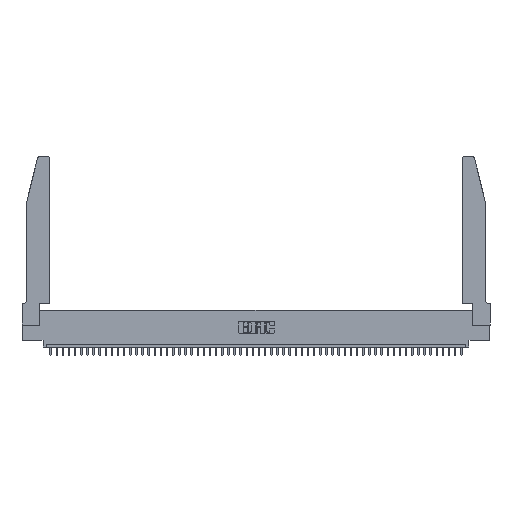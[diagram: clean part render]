
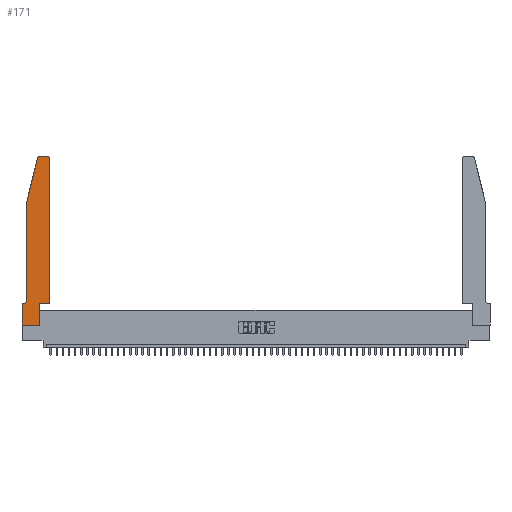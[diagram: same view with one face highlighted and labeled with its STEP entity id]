
A CAD part, top view. The second image highlights one B-rep face of the part: STEP entity #171.
In plain terms, the highlighted planar face has unit normal (0, 0, 1).
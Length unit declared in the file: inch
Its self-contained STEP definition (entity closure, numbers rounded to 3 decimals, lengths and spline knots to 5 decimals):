
#13 = ORIENTED_EDGE ( 'NONE', *, *, #20485, .T. ) ;
#171 = ADVANCED_FACE ( 'NONE', ( #5530 ), #13659, .T. ) ;
#1141 = ORIENTED_EDGE ( 'NONE', *, *, #18032, .T. ) ;
#1325 = CARTESIAN_POINT ( 'NONE',  ( 0., 0., 0.37 ) ) ;
#1405 = CARTESIAN_POINT ( 'NONE',  ( 0.2865, 0.35, 0.37 ) ) ;
#1880 = CARTESIAN_POINT ( 'NONE',  ( 0.4205, 2.75, 0.37 ) ) ;
#2229 = VECTOR ( 'NONE', #12704, 39.37008 ) ;
#2287 = CARTESIAN_POINT ( 'NONE',  ( 0.25487, 2.72718, 0.37 ) ) ;
#2716 = DIRECTION ( 'NONE',  ( 1., 0., 0. ) ) ;
#3330 = VECTOR ( 'NONE', #49036, 39.37008 ) ;
#3347 = EDGE_CURVE ( 'NONE', #30168, #31658, #4534, .T. ) ;
#4101 = LINE ( 'NONE', #18395, #52424 ) ;
#4330 = LINE ( 'NONE', #1405, #24577 ) ;
#4534 = LINE ( 'NONE', #32354, #3330 ) ;
#4567 = CARTESIAN_POINT ( 'NONE',  ( 0.0755, 0.42, 0.37 ) ) ;
#4757 = DIRECTION ( 'NONE',  ( 1., 0., 0. ) ) ;
#4932 = LINE ( 'NONE', #9479, #21395 ) ;
#5530 = FACE_OUTER_BOUND ( 'NONE', #16073, .T. ) ;
#5671 = CARTESIAN_POINT ( 'NONE',  ( 0., 0.35, 0.37 ) ) ;
#6887 = CARTESIAN_POINT ( 'NONE',  ( 0.4505, 0.35, 0.37 ) ) ;
#7756 = LINE ( 'NONE', #6887, #33646 ) ;
#8350 = AXIS2_PLACEMENT_3D ( 'NONE', #5671, #14010, #30314 ) ;
#8376 = CIRCLE ( 'NONE', #36357, 0.03 ) ;
#8532 = CARTESIAN_POINT ( 'NONE',  ( 0.4205, 2.72, 0.37 ) ) ;
#8862 = EDGE_CURVE ( 'NONE', #36129, #30168, #27700, .T. ) ;
#9057 = DIRECTION ( 'NONE',  ( 0., 0., -1. ) ) ;
#9324 = EDGE_CURVE ( 'NONE', #16800, #15200, #37878, .T. ) ;
#9479 = CARTESIAN_POINT ( 'NONE',  ( 0.4505, 0.35, 0.37 ) ) ;
#9498 = CARTESIAN_POINT ( 'NONE',  ( 0.284, 2.75, 0.37 ) ) ;
#9844 = CARTESIAN_POINT ( 'NONE',  ( 0., 0.35, 0.37 ) ) ;
#11796 = VERTEX_POINT ( 'NONE', #40973 ) ;
#12537 = CARTESIAN_POINT ( 'NONE',  ( 0.0755, 2., 0.37 ) ) ;
#12704 = DIRECTION ( 'NONE',  ( -0.239, -0.971, 0. ) ) ;
#12816 = EDGE_CURVE ( 'NONE', #49598, #34882, #16772, .T. ) ;
#13659 = PLANE ( 'NONE',  #8350 ) ;
#14010 = DIRECTION ( 'NONE',  ( 0., 0., 1. ) ) ;
#14015 = ORIENTED_EDGE ( 'NONE', *, *, #25178, .T. ) ;
#14162 = DIRECTION ( 'NONE',  ( 0., -1., 0. ) ) ;
#14476 = DIRECTION ( 'NONE',  ( 1., 0., 0. ) ) ;
#15200 = VERTEX_POINT ( 'NONE', #1880 ) ;
#15762 = CIRCLE ( 'NONE', #35798, 0.07 ) ;
#16073 = EDGE_LOOP ( 'NONE', ( #1141, #28969, #47659, #48011, #13, #52396, #35775, #38421, #27504, #38882, #14015, #41162 ) ) ;
#16536 = LINE ( 'NONE', #1325, #35635 ) ;
#16772 = LINE ( 'NONE', #12537, #2229 ) ;
#16800 = VERTEX_POINT ( 'NONE', #46149 ) ;
#17211 = EDGE_CURVE ( 'NONE', #19001, #30820, #4330, .T. ) ;
#18032 = EDGE_CURVE ( 'NONE', #15200, #28857, #52316, .T. ) ;
#18395 = CARTESIAN_POINT ( 'NONE',  ( 0.0755, 2., 0.37 ) ) ;
#19001 = VERTEX_POINT ( 'NONE', #19249 ) ;
#19249 = CARTESIAN_POINT ( 'NONE',  ( 0.2865, 0., 0.37 ) ) ;
#20126 = AXIS2_PLACEMENT_3D ( 'NONE', #8532, #29008, #4757 ) ;
#20485 = EDGE_CURVE ( 'NONE', #28073, #36129, #15762, .T. ) ;
#20636 = CARTESIAN_POINT ( 'NONE',  ( 0., 0., 0.37 ) ) ;
#21395 = VECTOR ( 'NONE', #50297, 39.37008 ) ;
#24577 = VECTOR ( 'NONE', #49690, 39.37008 ) ;
#25178 = EDGE_CURVE ( 'NONE', #11796, #16800, #4932, .T. ) ;
#25651 = CARTESIAN_POINT ( 'NONE',  ( 0.284, 2.72, 0.37 ) ) ;
#27504 = ORIENTED_EDGE ( 'NONE', *, *, #17211, .T. ) ;
#27700 = LINE ( 'NONE', #36387, #48770 ) ;
#27783 = DIRECTION ( 'NONE',  ( -1., 0., 0. ) ) ;
#28073 = VERTEX_POINT ( 'NONE', #4567 ) ;
#28617 = VECTOR ( 'NONE', #50097, 39.37008 ) ;
#28857 = VERTEX_POINT ( 'NONE', #9498 ) ;
#28969 = ORIENTED_EDGE ( 'NONE', *, *, #29483, .T. ) ;
#29008 = DIRECTION ( 'NONE',  ( 0., 0., 1. ) ) ;
#29483 = EDGE_CURVE ( 'NONE', #28857, #49598, #8376, .T. ) ;
#30168 = VERTEX_POINT ( 'NONE', #9844 ) ;
#30314 = DIRECTION ( 'NONE',  ( 1., 0., 0. ) ) ;
#30820 = VERTEX_POINT ( 'NONE', #33991 ) ;
#31658 = VERTEX_POINT ( 'NONE', #20636 ) ;
#32354 = CARTESIAN_POINT ( 'NONE',  ( 0., 0., 0.37 ) ) ;
#33321 = CARTESIAN_POINT ( 'NONE',  ( 0.0055, 0.42, 0.37 ) ) ;
#33646 = VECTOR ( 'NONE', #35231, 39.37008 ) ;
#33991 = CARTESIAN_POINT ( 'NONE',  ( 0.2865, 0.35, 0.37 ) ) ;
#34248 = EDGE_CURVE ( 'NONE', #34882, #28073, #4101, .T. ) ;
#34882 = VERTEX_POINT ( 'NONE', #36958 ) ;
#35231 = DIRECTION ( 'NONE',  ( 1., 0., 0. ) ) ;
#35635 = VECTOR ( 'NONE', #14476, 39.37008 ) ;
#35775 = ORIENTED_EDGE ( 'NONE', *, *, #3347, .T. ) ;
#35798 = AXIS2_PLACEMENT_3D ( 'NONE', #33321, #9057, #41549 ) ;
#36129 = VERTEX_POINT ( 'NONE', #39762 ) ;
#36357 = AXIS2_PLACEMENT_3D ( 'NONE', #25651, #42109, #2716 ) ;
#36387 = CARTESIAN_POINT ( 'NONE',  ( 0.0755, 0.35, 0.37 ) ) ;
#36958 = CARTESIAN_POINT ( 'NONE',  ( 0.0755, 2., 0.37 ) ) ;
#37878 = CIRCLE ( 'NONE', #20126, 0.03 ) ;
#37879 = CARTESIAN_POINT ( 'NONE',  ( 0.2605, 2.75, 0.37 ) ) ;
#38421 = ORIENTED_EDGE ( 'NONE', *, *, #42745, .T. ) ;
#38882 = ORIENTED_EDGE ( 'NONE', *, *, #51618, .T. ) ;
#39762 = CARTESIAN_POINT ( 'NONE',  ( 0.0055, 0.35, 0.37 ) ) ;
#40973 = CARTESIAN_POINT ( 'NONE',  ( 0.4505, 0.35, 0.37 ) ) ;
#41162 = ORIENTED_EDGE ( 'NONE', *, *, #9324, .T. ) ;
#41549 = DIRECTION ( 'NONE',  ( -1., 0., 0. ) ) ;
#42109 = DIRECTION ( 'NONE',  ( 0., 0., 1. ) ) ;
#42745 = EDGE_CURVE ( 'NONE', #31658, #19001, #16536, .T. ) ;
#46149 = CARTESIAN_POINT ( 'NONE',  ( 0.4505, 2.72, 0.37 ) ) ;
#47659 = ORIENTED_EDGE ( 'NONE', *, *, #12816, .T. ) ;
#48011 = ORIENTED_EDGE ( 'NONE', *, *, #34248, .T. ) ;
#48770 = VECTOR ( 'NONE', #27783, 39.37008 ) ;
#49036 = DIRECTION ( 'NONE',  ( 0., -1., 0. ) ) ;
#49598 = VERTEX_POINT ( 'NONE', #2287 ) ;
#49690 = DIRECTION ( 'NONE',  ( 0., 1., 0. ) ) ;
#50097 = DIRECTION ( 'NONE',  ( -1., 0., 0. ) ) ;
#50297 = DIRECTION ( 'NONE',  ( 0., 1., 0. ) ) ;
#51618 = EDGE_CURVE ( 'NONE', #30820, #11796, #7756, .T. ) ;
#52316 = LINE ( 'NONE', #37879, #28617 ) ;
#52396 = ORIENTED_EDGE ( 'NONE', *, *, #8862, .T. ) ;
#52424 = VECTOR ( 'NONE', #14162, 39.37008 ) ;
